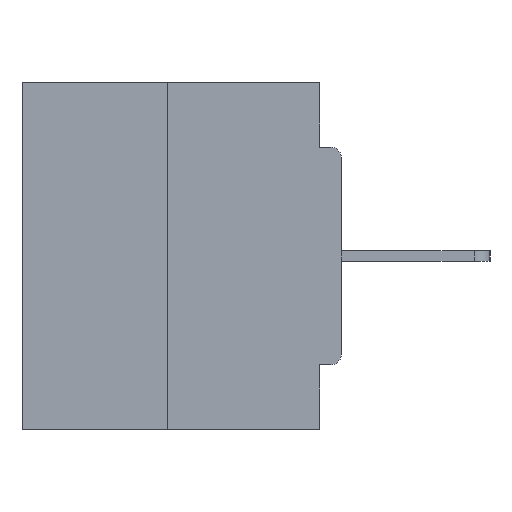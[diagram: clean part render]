
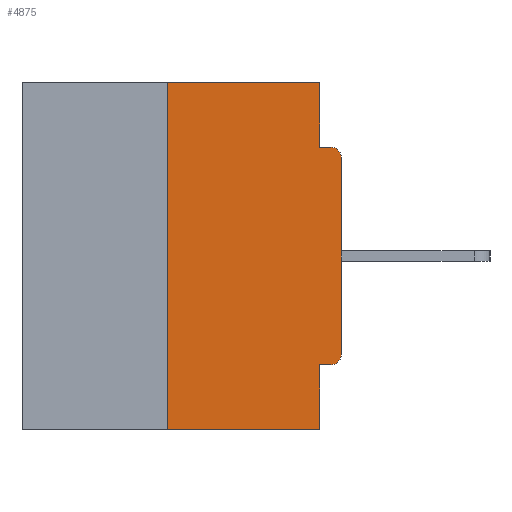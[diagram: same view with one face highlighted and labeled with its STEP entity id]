
A CAD part, left-side view. The second image highlights one B-rep face of the part: STEP entity #4875.
In plain terms, the highlighted planar face has unit normal (-1, 0, 0).
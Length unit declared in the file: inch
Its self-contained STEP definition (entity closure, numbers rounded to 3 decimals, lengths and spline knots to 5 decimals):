
#128 = ORIENTED_EDGE ( 'NONE', *, *, #2099, .F. ) ;
#229 = EDGE_CURVE ( 'NONE', #15592, #14504, #2199, .T. ) ;
#295 = CARTESIAN_POINT ( 'NONE',  ( 0., 0., -0.0935 ) ) ;
#505 = EDGE_CURVE ( 'NONE', #13823, #22955, #26913, .T. ) ;
#632 = VECTOR ( 'NONE', #23817, 39.37008 ) ;
#730 = VERTEX_POINT ( 'NONE', #16082 ) ;
#1044 = VECTOR ( 'NONE', #8397, 39.37008 ) ;
#2099 = EDGE_CURVE ( 'NONE', #14504, #15546, #13581, .T. ) ;
#2199 = LINE ( 'NONE', #3211, #8727 ) ;
#2427 = CARTESIAN_POINT ( 'NONE',  ( 0., 0.46, 0. ) ) ;
#2436 = CARTESIAN_POINT ( 'NONE',  ( 0., 0.25, 0. ) ) ;
#2645 = DIRECTION ( 'NONE',  ( 0., 0., -1. ) ) ;
#2982 = ORIENTED_EDGE ( 'NONE', *, *, #505, .F. ) ;
#3211 = CARTESIAN_POINT ( 'NONE',  ( 0., 0.46, 0. ) ) ;
#4208 = LINE ( 'NONE', #295, #22920 ) ;
#4561 = VERTEX_POINT ( 'NONE', #18356 ) ;
#4875 = ADVANCED_FACE ( 'NONE', ( #27683 ), #19597, .F. ) ;
#5244 = CARTESIAN_POINT ( 'NONE',  ( 0., 0.25, 0. ) ) ;
#5691 = AXIS2_PLACEMENT_3D ( 'NONE', #12615, #29493, #15091 ) ;
#6146 = DIRECTION ( 'NONE',  ( 0., 0., -1. ) ) ;
#6281 = CARTESIAN_POINT ( 'NONE',  ( 0., 0.015, -0.1085 ) ) ;
#7053 = CARTESIAN_POINT ( 'NONE',  ( 0., 0.031, 0. ) ) ;
#7165 = LINE ( 'NONE', #21430, #632 ) ;
#7201 = LINE ( 'NONE', #17363, #26563 ) ;
#7377 = DIRECTION ( 'NONE',  ( 0., 0., -1. ) ) ;
#7750 = AXIS2_PLACEMENT_3D ( 'NONE', #6281, #23331, #8750 ) ;
#8298 = ORIENTED_EDGE ( 'NONE', *, *, #9736, .T. ) ;
#8397 = DIRECTION ( 'NONE',  ( 0., 1., 0. ) ) ;
#8451 = DIRECTION ( 'NONE',  ( 0., -1., 0. ) ) ;
#8601 = EDGE_LOOP ( 'NONE', ( #19190, #11985, #13258, #14538, #2982, #8298, #13157, #19790, #21355, #128 ) ) ;
#8727 = VECTOR ( 'NONE', #8451, 39.37008 ) ;
#8750 = DIRECTION ( 'NONE',  ( 0., 0., -1. ) ) ;
#8803 = DIRECTION ( 'NONE',  ( 0., -1., 0. ) ) ;
#9736 = EDGE_CURVE ( 'NONE', #13823, #4561, #13425, .T. ) ;
#11256 = CARTESIAN_POINT ( 'NONE',  ( 0., 0., -0.4065 ) ) ;
#11326 = CARTESIAN_POINT ( 'NONE',  ( 0., 0.015, -0.0935 ) ) ;
#11985 = ORIENTED_EDGE ( 'NONE', *, *, #30996, .F. ) ;
#12615 = CARTESIAN_POINT ( 'NONE',  ( 0., 0.015, -0.3915 ) ) ;
#12944 = LINE ( 'NONE', #16199, #19486 ) ;
#13157 = ORIENTED_EDGE ( 'NONE', *, *, #16102, .T. ) ;
#13258 = ORIENTED_EDGE ( 'NONE', *, *, #30638, .T. ) ;
#13425 = CIRCLE ( 'NONE', #5691, 0.015 ) ;
#13581 = LINE ( 'NONE', #7053, #20841 ) ;
#13670 = CARTESIAN_POINT ( 'NONE',  ( 0., 0.031, -0.5 ) ) ;
#13823 = VERTEX_POINT ( 'NONE', #20346 ) ;
#14504 = VERTEX_POINT ( 'NONE', #20408 ) ;
#14538 = ORIENTED_EDGE ( 'NONE', *, *, #15648, .F. ) ;
#14549 = CARTESIAN_POINT ( 'NONE',  ( 0., 0.031, -0.0935 ) ) ;
#15091 = DIRECTION ( 'NONE',  ( 0., 0., -1. ) ) ;
#15546 = VERTEX_POINT ( 'NONE', #14549 ) ;
#15592 = VERTEX_POINT ( 'NONE', #2436 ) ;
#15648 = EDGE_CURVE ( 'NONE', #22955, #18526, #7201, .T. ) ;
#16082 = CARTESIAN_POINT ( 'NONE',  ( 0., 0., -0.1085 ) ) ;
#16102 = EDGE_CURVE ( 'NONE', #4561, #730, #7165, .T. ) ;
#16199 = CARTESIAN_POINT ( 'NONE',  ( 0., 0.46, -0.5 ) ) ;
#17363 = CARTESIAN_POINT ( 'NONE',  ( 0., 0.031, -0.5 ) ) ;
#17927 = CARTESIAN_POINT ( 'NONE',  ( 0., 0.25, -0.5 ) ) ;
#18356 = CARTESIAN_POINT ( 'NONE',  ( 0., 0., -0.3915 ) ) ;
#18526 = VERTEX_POINT ( 'NONE', #13670 ) ;
#19190 = ORIENTED_EDGE ( 'NONE', *, *, #229, .F. ) ;
#19486 = VECTOR ( 'NONE', #8803, 39.37008 ) ;
#19597 = PLANE ( 'NONE',  #27556 ) ;
#19790 = ORIENTED_EDGE ( 'NONE', *, *, #20291, .T. ) ;
#20291 = EDGE_CURVE ( 'NONE', #730, #27792, #28125, .T. ) ;
#20346 = CARTESIAN_POINT ( 'NONE',  ( 0., 0.015, -0.4065 ) ) ;
#20408 = CARTESIAN_POINT ( 'NONE',  ( 0., 0.031, 0. ) ) ;
#20841 = VECTOR ( 'NONE', #6146, 39.37008 ) ;
#20944 = VECTOR ( 'NONE', #24619, 39.37008 ) ;
#21355 = ORIENTED_EDGE ( 'NONE', *, *, #23015, .F. ) ;
#21430 = CARTESIAN_POINT ( 'NONE',  ( 0., 0., 0. ) ) ;
#21979 = DIRECTION ( 'NONE',  ( 1., 0., 0. ) ) ;
#22920 = VECTOR ( 'NONE', #27106, 39.37008 ) ;
#22955 = VERTEX_POINT ( 'NONE', #29199 ) ;
#23015 = EDGE_CURVE ( 'NONE', #15546, #27792, #4208, .T. ) ;
#23331 = DIRECTION ( 'NONE',  ( -1., 0., 0. ) ) ;
#23817 = DIRECTION ( 'NONE',  ( 0., 0., 1. ) ) ;
#24619 = DIRECTION ( 'NONE',  ( 0., 0., 1. ) ) ;
#25689 = VERTEX_POINT ( 'NONE', #17927 ) ;
#26563 = VECTOR ( 'NONE', #2645, 39.37008 ) ;
#26913 = LINE ( 'NONE', #11256, #1044 ) ;
#27106 = DIRECTION ( 'NONE',  ( 0., -1., 0. ) ) ;
#27284 = LINE ( 'NONE', #5244, #20944 ) ;
#27556 = AXIS2_PLACEMENT_3D ( 'NONE', #2427, #21979, #7377 ) ;
#27683 = FACE_OUTER_BOUND ( 'NONE', #8601, .T. ) ;
#27792 = VERTEX_POINT ( 'NONE', #11326 ) ;
#28125 = CIRCLE ( 'NONE', #7750, 0.015 ) ;
#29199 = CARTESIAN_POINT ( 'NONE',  ( 0., 0.031, -0.4065 ) ) ;
#29493 = DIRECTION ( 'NONE',  ( -1., 0., 0. ) ) ;
#30638 = EDGE_CURVE ( 'NONE', #25689, #18526, #12944, .T. ) ;
#30996 = EDGE_CURVE ( 'NONE', #25689, #15592, #27284, .T. ) ;
